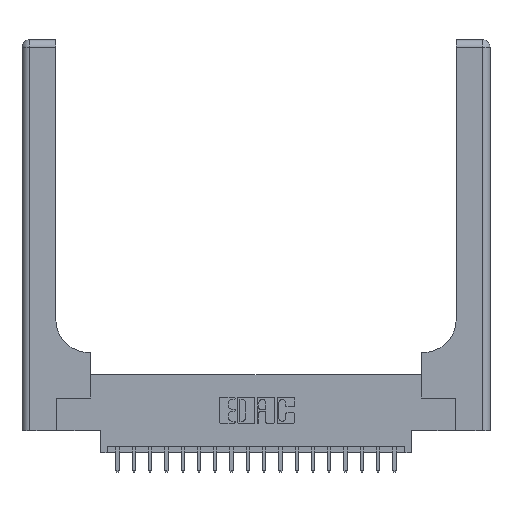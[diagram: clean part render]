
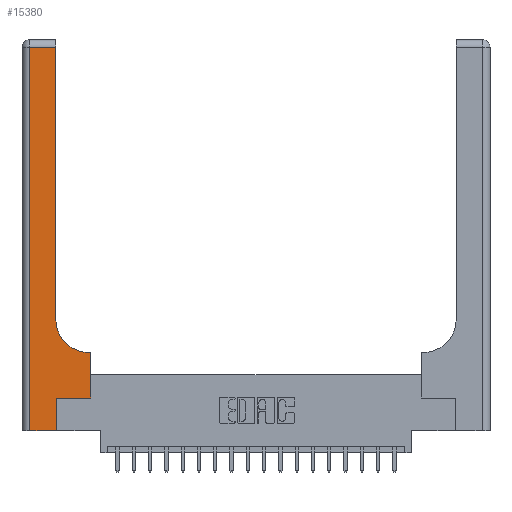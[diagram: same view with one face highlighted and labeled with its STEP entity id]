
A CAD part, top view. The second image highlights one B-rep face of the part: STEP entity #15380.
In plain terms, the highlighted planar face has unit normal (0, 0, 1).
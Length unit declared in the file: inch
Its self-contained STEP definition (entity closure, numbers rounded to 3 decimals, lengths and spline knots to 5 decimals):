
#10 = DIRECTION ( 'NONE',  ( -1., 0., 0. ) ) ;
#169 = DIRECTION ( 'NONE',  ( -1., 0., 0. ) ) ;
#881 = AXIS2_PLACEMENT_3D ( 'NONE', #4214, #15200, #5827 ) ;
#1398 = DIRECTION ( 'NONE',  ( 1., 0., 0. ) ) ;
#2130 = VECTOR ( 'NONE', #169, 39.37008 ) ;
#2259 = CARTESIAN_POINT ( 'NONE',  ( 0.528, 0.6, 0.37 ) ) ;
#2313 = CARTESIAN_POINT ( 'NONE',  ( 0.51, 0.6, 0.37 ) ) ;
#2750 = ORIENTED_EDGE ( 'NONE', *, *, #3303, .T. ) ;
#2921 = CARTESIAN_POINT ( 'NONE',  ( 0.528, 0.25, 0.37 ) ) ;
#3109 = VERTEX_POINT ( 'NONE', #11921 ) ;
#3159 = LINE ( 'NONE', #18910, #15245 ) ;
#3303 = EDGE_CURVE ( 'NONE', #20309, #13925, #18102, .T. ) ;
#4141 = PLANE ( 'NONE',  #881 ) ;
#4214 = CARTESIAN_POINT ( 'NONE',  ( 0., 3., 0.37 ) ) ;
#4300 = EDGE_CURVE ( 'NONE', #8890, #18594, #18065, .T. ) ;
#4575 = DIRECTION ( 'NONE',  ( 0., 1., 0. ) ) ;
#4584 = EDGE_LOOP ( 'NONE', ( #14654, #16223, #2750, #16527, #15964, #16130, #11248, #12351, #14969 ) ) ;
#4702 = LINE ( 'NONE', #6000, #12540 ) ;
#4824 = CIRCLE ( 'NONE', #9992, 0.25 ) ;
#4863 = VERTEX_POINT ( 'NONE', #2313 ) ;
#5036 = CARTESIAN_POINT ( 'NONE',  ( 0.265, 0., 0.37 ) ) ;
#5749 = EDGE_CURVE ( 'NONE', #4863, #15952, #4824, .T. ) ;
#5827 = DIRECTION ( 'NONE',  ( -1., 0., 0. ) ) ;
#5989 = DIRECTION ( 'NONE',  ( 1., 0., 0. ) ) ;
#6000 = CARTESIAN_POINT ( 'NONE',  ( 0.26, 3., 0.37 ) ) ;
#6027 = CARTESIAN_POINT ( 'NONE',  ( 0.265, 0., 0.37 ) ) ;
#6275 = EDGE_CURVE ( 'NONE', #8219, #15234, #19852, .T. ) ;
#6508 = DIRECTION ( 'NONE',  ( 0., 0., -1. ) ) ;
#8219 = VERTEX_POINT ( 'NONE', #13810 ) ;
#8422 = FACE_OUTER_BOUND ( 'NONE', #4584, .T. ) ;
#8890 = VERTEX_POINT ( 'NONE', #6027 ) ;
#8932 = CARTESIAN_POINT ( 'NONE',  ( 0.26, 0.85, 0.37 ) ) ;
#9478 = EDGE_CURVE ( 'NONE', #15952, #3109, #4702, .T. ) ;
#9773 = VECTOR ( 'NONE', #11338, 39.37008 ) ;
#9811 = VECTOR ( 'NONE', #10731, 39.37008 ) ;
#9992 = AXIS2_PLACEMENT_3D ( 'NONE', #15819, #6508, #17381 ) ;
#10592 = EDGE_CURVE ( 'NONE', #18594, #8219, #19273, .T. ) ;
#10731 = DIRECTION ( 'NONE',  ( 0., -1., 0. ) ) ;
#11248 = ORIENTED_EDGE ( 'NONE', *, *, #6275, .T. ) ;
#11338 = DIRECTION ( 'NONE',  ( 0., 1., 0. ) ) ;
#11921 = CARTESIAN_POINT ( 'NONE',  ( 0.26, 2.94, 0.37 ) ) ;
#12217 = CARTESIAN_POINT ( 'NONE',  ( 0.265, 0.25, 0.37 ) ) ;
#12351 = ORIENTED_EDGE ( 'NONE', *, *, #19471, .T. ) ;
#12540 = VECTOR ( 'NONE', #15360, 39.37008 ) ;
#13810 = CARTESIAN_POINT ( 'NONE',  ( 0.528, 0.25, 0.37 ) ) ;
#13925 = VERTEX_POINT ( 'NONE', #19399 ) ;
#14008 = VECTOR ( 'NONE', #5989, 39.37008 ) ;
#14205 = CARTESIAN_POINT ( 'NONE',  ( 0.06, 2.94, 0.37 ) ) ;
#14654 = ORIENTED_EDGE ( 'NONE', *, *, #9478, .T. ) ;
#14701 = VECTOR ( 'NONE', #1398, 39.37008 ) ;
#14768 = LINE ( 'NONE', #19052, #2130 ) ;
#14969 = ORIENTED_EDGE ( 'NONE', *, *, #5749, .T. ) ;
#15200 = DIRECTION ( 'NONE',  ( 0., 0., -1. ) ) ;
#15234 = VERTEX_POINT ( 'NONE', #2259 ) ;
#15245 = VECTOR ( 'NONE', #10, 39.37008 ) ;
#15360 = DIRECTION ( 'NONE',  ( 0., 1., 0. ) ) ;
#15380 = ADVANCED_FACE ( 'NONE', ( #8422 ), #4141, .F. ) ;
#15819 = CARTESIAN_POINT ( 'NONE',  ( 0.51, 0.85, 0.37 ) ) ;
#15952 = VERTEX_POINT ( 'NONE', #8932 ) ;
#15964 = ORIENTED_EDGE ( 'NONE', *, *, #4300, .T. ) ;
#16130 = ORIENTED_EDGE ( 'NONE', *, *, #10592, .T. ) ;
#16223 = ORIENTED_EDGE ( 'NONE', *, *, #19872, .T. ) ;
#16527 = ORIENTED_EDGE ( 'NONE', *, *, #18608, .T. ) ;
#17381 = DIRECTION ( 'NONE',  ( 1., 0., 0. ) ) ;
#18065 = LINE ( 'NONE', #5036, #9773 ) ;
#18102 = LINE ( 'NONE', #19972, #9811 ) ;
#18159 = LINE ( 'NONE', #18454, #14008 ) ;
#18454 = CARTESIAN_POINT ( 'NONE',  ( 0., 0., 0.37 ) ) ;
#18594 = VERTEX_POINT ( 'NONE', #12217 ) ;
#18608 = EDGE_CURVE ( 'NONE', #13925, #8890, #18159, .T. ) ;
#18910 = CARTESIAN_POINT ( 'NONE',  ( 0., 2.94, 0.37 ) ) ;
#19052 = CARTESIAN_POINT ( 'NONE',  ( 0.26, 0.6, 0.37 ) ) ;
#19273 = LINE ( 'NONE', #20170, #14701 ) ;
#19397 = VECTOR ( 'NONE', #4575, 39.37008 ) ;
#19399 = CARTESIAN_POINT ( 'NONE',  ( 0.06, 0., 0.37 ) ) ;
#19471 = EDGE_CURVE ( 'NONE', #15234, #4863, #14768, .T. ) ;
#19852 = LINE ( 'NONE', #2921, #19397 ) ;
#19872 = EDGE_CURVE ( 'NONE', #3109, #20309, #3159, .T. ) ;
#19972 = CARTESIAN_POINT ( 'NONE',  ( 0.06, 3., 0.37 ) ) ;
#20170 = CARTESIAN_POINT ( 'NONE',  ( 0.265, 0.25, 0.37 ) ) ;
#20309 = VERTEX_POINT ( 'NONE', #14205 ) ;
